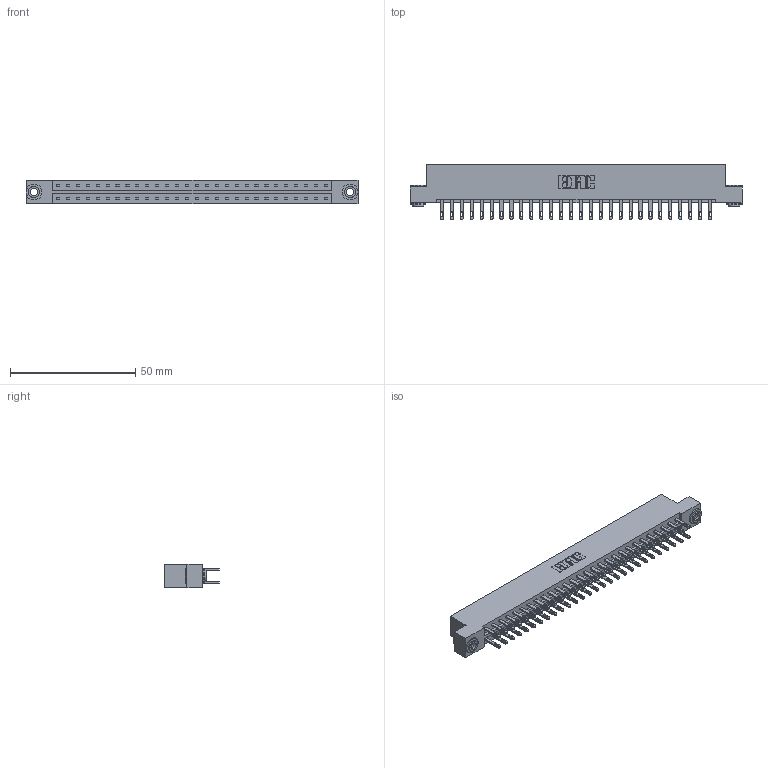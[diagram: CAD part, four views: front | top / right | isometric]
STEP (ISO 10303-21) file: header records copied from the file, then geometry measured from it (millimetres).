
FILE_DESCRIPTION (( 'STEP AP203' ), '1' );
FILE_NAME ('833-056-500-203.STEP', '2020-06-04T22:00:05', ( '' ), ( '' ), 'SwSTEP 2.0', 'SolidWorks 2020', '' );
FILE_SCHEMA (( 'CONFIG_CONTROL_DESIGN' ));
Length unit declared in the file: inch
Products named in the file (4): 345-292-001_345-293-100; 345-250-002_345-250-002-102; 833 Part_Flush - .156 Dia - TH; 833-056-500-203
Assembly tree (59 placements, depth 2):
  833-056-500-203
    833 Part_Flush - .156 Dia - TH
    345-292-001_345-293-100  x56
    345-250-002_345-250-002-102  x2
Bounding box: 132.49 x 21.85 x 9.4 mm (x, y, z)
Volume: 13585.7 mm3; surface area: 16748.4 mm2
Topology: 59 solids, 59 shells, 2840 faces, 8619 edges, 5742 vertices
Faces by surface type: plane 1760, cylinder 1072, cone 8
Entity records: 20404 total; most frequent: CARTESIAN_POINT 3373, ORIENTED_EDGE 3302, DIRECTION 2941, EDGE_CURVE 1651, LINE 1495, VECTOR 1495, VERTEX_POINT 1098, AXIS2_PLACEMENT_3D 723
